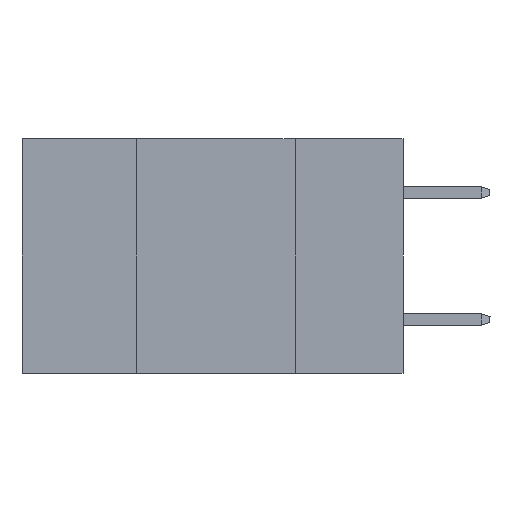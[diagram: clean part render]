
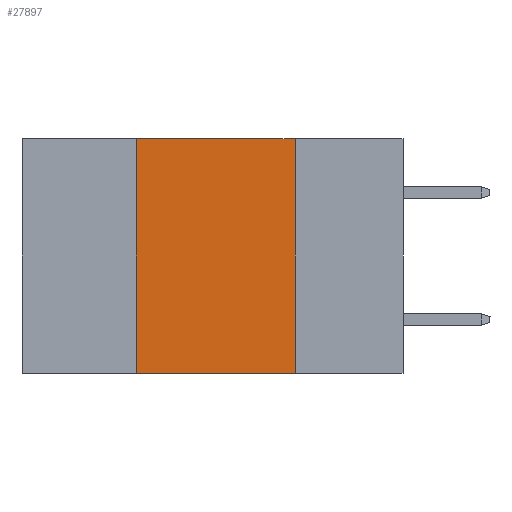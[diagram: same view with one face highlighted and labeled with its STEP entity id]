
A CAD part, left-side view. The second image highlights one B-rep face of the part: STEP entity #27897.
In plain terms, the highlighted planar face has unit normal (-1, 0, 0).
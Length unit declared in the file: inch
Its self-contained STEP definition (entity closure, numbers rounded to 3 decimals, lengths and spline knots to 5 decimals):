
#1265 = DIRECTION ( 'NONE',  ( 0., -1., 0. ) ) ;
#1759 = LINE ( 'NONE', #4156, #16166 ) ;
#4156 = CARTESIAN_POINT ( 'NONE',  ( 0., 0.6, 0. ) ) ;
#4638 = ORIENTED_EDGE ( 'NONE', *, *, #24029, .F. ) ;
#5237 = DIRECTION ( 'NONE',  ( 1., 0., 0. ) ) ;
#5774 = VECTOR ( 'NONE', #9933, 39.37008 ) ;
#6929 = VECTOR ( 'NONE', #11191, 39.37008 ) ;
#7357 = CARTESIAN_POINT ( 'NONE',  ( 0., 0.6, 0. ) ) ;
#7926 = CARTESIAN_POINT ( 'NONE',  ( 0., 0.42, -0.37 ) ) ;
#7943 = ORIENTED_EDGE ( 'NONE', *, *, #17702, .F. ) ;
#8184 = CARTESIAN_POINT ( 'NONE',  ( 0., 0.6, -0.37 ) ) ;
#9752 = VERTEX_POINT ( 'NONE', #22933 ) ;
#9933 = DIRECTION ( 'NONE',  ( 0., 0., -1. ) ) ;
#9951 = VECTOR ( 'NONE', #1265, 39.37008 ) ;
#10278 = DIRECTION ( 'NONE',  ( 0., -1., 0. ) ) ;
#10334 = LINE ( 'NONE', #8184, #9951 ) ;
#11107 = VERTEX_POINT ( 'NONE', #17560 ) ;
#11191 = DIRECTION ( 'NONE',  ( 0., 0., 1. ) ) ;
#11503 = EDGE_CURVE ( 'NONE', #25299, #11107, #10334, .T. ) ;
#12196 = LINE ( 'NONE', #18540, #5774 ) ;
#12618 = AXIS2_PLACEMENT_3D ( 'NONE', #7357, #5237, #22521 ) ;
#14617 = ORIENTED_EDGE ( 'NONE', *, *, #11503, .T. ) ;
#15014 = CARTESIAN_POINT ( 'NONE',  ( 0., 0.42, 0. ) ) ;
#16166 = VECTOR ( 'NONE', #10278, 39.37008 ) ;
#17143 = ORIENTED_EDGE ( 'NONE', *, *, #24481, .F. ) ;
#17560 = CARTESIAN_POINT ( 'NONE',  ( 0., 0.17, -0.37 ) ) ;
#17702 = EDGE_CURVE ( 'NONE', #25299, #22883, #20380, .T. ) ;
#18540 = CARTESIAN_POINT ( 'NONE',  ( 0., 0.17, 0. ) ) ;
#20230 = CARTESIAN_POINT ( 'NONE',  ( 0., 0.42, 0. ) ) ;
#20238 = PLANE ( 'NONE',  #12618 ) ;
#20380 = LINE ( 'NONE', #20230, #6929 ) ;
#21942 = EDGE_LOOP ( 'NONE', ( #4638, #17143, #7943, #14617 ) ) ;
#22521 = DIRECTION ( 'NONE',  ( 0., 0., -1. ) ) ;
#22883 = VERTEX_POINT ( 'NONE', #15014 ) ;
#22933 = CARTESIAN_POINT ( 'NONE',  ( 0., 0.17, 0. ) ) ;
#24029 = EDGE_CURVE ( 'NONE', #9752, #11107, #12196, .T. ) ;
#24481 = EDGE_CURVE ( 'NONE', #22883, #9752, #1759, .T. ) ;
#24521 = FACE_OUTER_BOUND ( 'NONE', #21942, .T. ) ;
#25299 = VERTEX_POINT ( 'NONE', #7926 ) ;
#27897 = ADVANCED_FACE ( 'NONE', ( #24521 ), #20238, .F. ) ;
